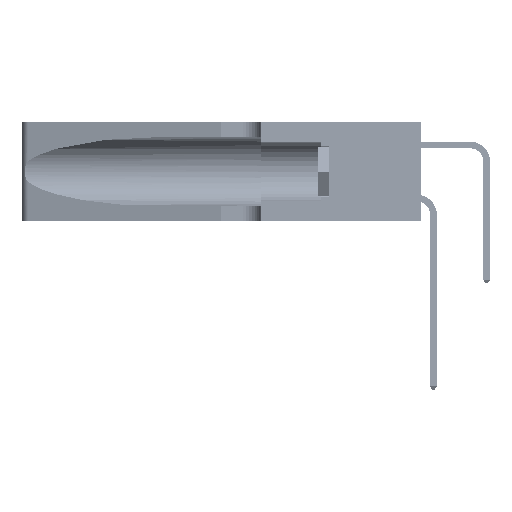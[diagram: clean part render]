
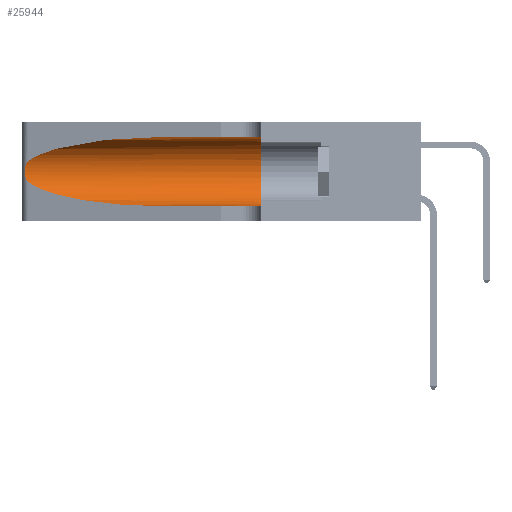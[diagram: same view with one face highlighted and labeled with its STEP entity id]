
A CAD part, left-side view. The second image highlights one B-rep face of the part: STEP entity #25944.
In plain terms, the highlighted cylindrical face has radius 3.308 mm (diameter 6.617 mm), a partial arc.
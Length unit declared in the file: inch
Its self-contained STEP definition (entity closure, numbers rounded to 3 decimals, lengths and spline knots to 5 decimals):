
#628 = VERTEX_POINT ( 'NONE', #28994 ) ;
#1496 =( BOUNDED_CURVE ( )  B_SPLINE_CURVE ( 3, ( #42767, #29272, #12891, #16631 ),
 .UNSPECIFIED., .F., .F. ) 
 B_SPLINE_CURVE_WITH_KNOTS ( ( 4, 4 ),
 ( 3.44316, 4.71239 ),
 .UNSPECIFIED. ) 
 CURVE ( )  GEOMETRIC_REPRESENTATION_ITEM ( )  RATIONAL_B_SPLINE_CURVE ( ( 1., 0.87, 0.87, 1. ) ) 
 REPRESENTATION_ITEM ( '' )  );
#2083 = CARTESIAN_POINT ( 'NONE',  ( 0.1305, 1.61858, 0.05475 ) ) ;
#3006 = CARTESIAN_POINT ( 'NONE',  ( 0.25787, 1.23484, 0.2124 ) ) ;
#3186 = CARTESIAN_POINT ( 'NONE',  ( 0.25639, 1.23184, 0.21858 ) ) ;
#3299 = CARTESIAN_POINT ( 'NONE',  ( 0.1305, 0.35, 0.31525 ) ) ;
#5040 = EDGE_CURVE ( 'NONE', #628, #10271, #49178, .T. ) ;
#5507 = ORIENTED_EDGE ( 'NONE', *, *, #18668, .F. ) ;
#7236 = CARTESIAN_POINT ( 'NONE',  ( 0.26018, 1.23835, 0.19895 ) ) ;
#7777 = CARTESIAN_POINT ( 'NONE',  ( 0.26017, 1.23833, 0.17102 ) ) ;
#8442 = CARTESIAN_POINT ( 'NONE',  ( 0.1305, 0.35, 0.05475 ) ) ;
#8666 = AXIS2_PLACEMENT_3D ( 'NONE', #20732, #20551, #50554 ) ;
#8787 = CARTESIAN_POINT ( 'NONE',  ( 0.18966, 0.96281, 0.31525 ) ) ;
#10271 = VERTEX_POINT ( 'NONE', #32471 ) ;
#11544 = CARTESIAN_POINT ( 'NONE',  ( 0.25856, 1.23593, 0.16098 ) ) ;
#11914 = ORIENTED_EDGE ( 'NONE', *, *, #47500, .T. ) ;
#12891 = CARTESIAN_POINT ( 'NONE',  ( 0.18966, 0.96281, 0.05475 ) ) ;
#13655 = VECTOR ( 'NONE', #40726, 39.37008 ) ;
#15479 = CARTESIAN_POINT ( 'NONE',  ( 0.25854, 1.2359, 0.20912 ) ) ;
#16631 = CARTESIAN_POINT ( 'NONE',  ( 0.1305, 0.72297, 0.05475 ) ) ;
#17687 = CIRCLE ( 'NONE', #26873, 0.13025 ) ;
#18668 = EDGE_CURVE ( 'NONE', #46887, #50254, #35239, .T. ) ;
#20313 = CARTESIAN_POINT ( 'NONE',  ( 0.26075, 1.23896, 0.178 ) ) ;
#20551 = DIRECTION ( 'NONE',  ( 0., -1., 0. ) ) ;
#20732 = CARTESIAN_POINT ( 'NONE',  ( 0.1305, 1.61858, 0.185 ) ) ;
#21678 = CARTESIAN_POINT ( 'NONE',  ( 0.1305, 0.72297, 0.31525 ) ) ;
#23726 =( BOUNDED_CURVE ( )  B_SPLINE_CURVE ( 3, ( #21678, #8787, #25578, #38544 ),
 .UNSPECIFIED., .F., .T. ) 
 B_SPLINE_CURVE_WITH_KNOTS ( ( 4, 4 ),
 ( 1.5708, 2.84003 ),
 .UNSPECIFIED. ) 
 CURVE ( )  GEOMETRIC_REPRESENTATION_ITEM ( )  RATIONAL_B_SPLINE_CURVE ( ( 1., 0.87, 0.87, 1. ) ) 
 REPRESENTATION_ITEM ( '' )  );
#24508 = EDGE_LOOP ( 'NONE', ( #33922, #29424, #11914, #27178, #40067, #5507 ) ) ;
#25578 = CARTESIAN_POINT ( 'NONE',  ( 0.2373, 1.15595, 0.28018 ) ) ;
#25944 = ADVANCED_FACE ( 'NONE', ( #46037 ), #46713, .F. ) ;
#26413 = EDGE_CURVE ( 'NONE', #50254, #53792, #17687, .T. ) ;
#26873 = AXIS2_PLACEMENT_3D ( 'NONE', #39971, #28293, #53470 ) ;
#27178 = ORIENTED_EDGE ( 'NONE', *, *, #37722, .T. ) ;
#28293 = DIRECTION ( 'NONE',  ( 0., 1., 0. ) ) ;
#28305 = CARTESIAN_POINT ( 'NONE',  ( 0.25487, 1.22718, 0.14631 ) ) ;
#28994 = CARTESIAN_POINT ( 'NONE',  ( 0.25487, 1.22718, 0.22369 ) ) ;
#29272 = CARTESIAN_POINT ( 'NONE',  ( 0.2373, 1.15595, 0.08982 ) ) ;
#29330 = CARTESIAN_POINT ( 'NONE',  ( 0.1305, 1.61858, 0.31525 ) ) ;
#29424 = ORIENTED_EDGE ( 'NONE', *, *, #5040, .T. ) ;
#32471 = CARTESIAN_POINT ( 'NONE',  ( 0.25487, 1.22718, 0.14631 ) ) ;
#33922 = ORIENTED_EDGE ( 'NONE', *, *, #39307, .T. ) ;
#35239 = LINE ( 'NONE', #29330, #37224 ) ;
#36275 = LINE ( 'NONE', #2083, #13655 ) ;
#36385 = CARTESIAN_POINT ( 'NONE',  ( 0.1305, 0.72297, 0.31525 ) ) ;
#37025 = CARTESIAN_POINT ( 'NONE',  ( 0.1305, 0.72297, 0.05475 ) ) ;
#37027 = CARTESIAN_POINT ( 'NONE',  ( 0.25555, 1.22994, 0.2215 ) ) ;
#37224 = VECTOR ( 'NONE', #42091, 39.37008 ) ;
#37722 = EDGE_CURVE ( 'NONE', #37899, #53792, #36275, .T. ) ;
#37899 = VERTEX_POINT ( 'NONE', #37025 ) ;
#38544 = CARTESIAN_POINT ( 'NONE',  ( 0.25487, 1.22718, 0.22369 ) ) ;
#39307 = EDGE_CURVE ( 'NONE', #46887, #628, #23726, .T. ) ;
#39971 = CARTESIAN_POINT ( 'NONE',  ( 0.1305, 0.35, 0.185 ) ) ;
#40067 = ORIENTED_EDGE ( 'NONE', *, *, #26413, .F. ) ;
#40726 = DIRECTION ( 'NONE',  ( 0., -1., 0. ) ) ;
#41271 = CARTESIAN_POINT ( 'NONE',  ( 0.25555, 1.22993, 0.14849 ) ) ;
#42091 = DIRECTION ( 'NONE',  ( 0., -1., 0. ) ) ;
#42767 = CARTESIAN_POINT ( 'NONE',  ( 0.25487, 1.22718, 0.14631 ) ) ;
#45175 = CARTESIAN_POINT ( 'NONE',  ( 0.25789, 1.23486, 0.15765 ) ) ;
#45713 = CARTESIAN_POINT ( 'NONE',  ( 0.25487, 1.22718, 0.22369 ) ) ;
#46037 = FACE_OUTER_BOUND ( 'NONE', #24508, .T. ) ;
#46713 = CYLINDRICAL_SURFACE ( 'NONE', #8666, 0.13025 ) ;
#46887 = VERTEX_POINT ( 'NONE', #36385 ) ;
#47500 = EDGE_CURVE ( 'NONE', #10271, #37899, #1496, .T. ) ;
#49178 = B_SPLINE_CURVE_WITH_KNOTS ( 'NONE', 3,
 ( #45713, #37027, #3186, #3006, #15479, #7236, #53667, #20313, #7777, #11544, #45175, #49967, #41271, #28305 ),
 .UNSPECIFIED., .F., .F.,
 ( 4, 2, 2, 2, 2, 2, 4 ),
 ( 0., 0.00027, 0.00053, 0.00107, 0.0016, 0.00187, 0.00214 ),
 .UNSPECIFIED. ) ;
#49967 = CARTESIAN_POINT ( 'NONE',  ( 0.25639, 1.23186, 0.15144 ) ) ;
#50254 = VERTEX_POINT ( 'NONE', #3299 ) ;
#50554 = DIRECTION ( 'NONE',  ( 0., 0., -1. ) ) ;
#53470 = DIRECTION ( 'NONE',  ( 0., 0., 1. ) ) ;
#53667 = CARTESIAN_POINT ( 'NONE',  ( 0.26075, 1.23896, 0.19203 ) ) ;
#53792 = VERTEX_POINT ( 'NONE', #8442 ) ;
